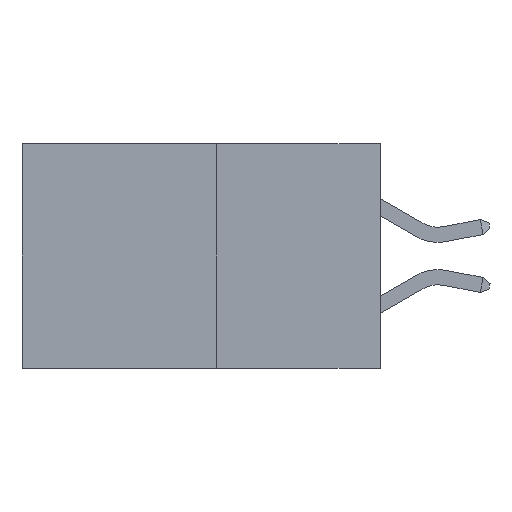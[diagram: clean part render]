
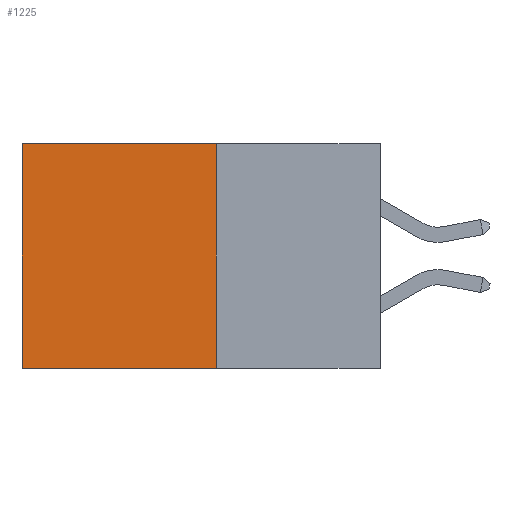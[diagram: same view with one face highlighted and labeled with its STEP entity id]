
A CAD part, left-side view. The second image highlights one B-rep face of the part: STEP entity #1225.
In plain terms, the highlighted planar face has unit normal (-1, 0, 0).
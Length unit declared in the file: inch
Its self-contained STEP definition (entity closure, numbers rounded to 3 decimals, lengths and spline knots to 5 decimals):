
#675 = CARTESIAN_POINT ( 'NONE',  ( 0.277, 0.59, -0.37 ) ) ;
#767 = LINE ( 'NONE', #675, #10291 ) ;
#862 = CARTESIAN_POINT ( 'NONE',  ( 0.277, 0.59, -0.37 ) ) ;
#999 = DIRECTION ( 'NONE',  ( 0., 1., 0. ) ) ;
#1225 = ADVANCED_FACE ( 'NONE', ( #3927 ), #4560, .F. ) ;
#1863 = CARTESIAN_POINT ( 'NONE',  ( 0.277, 0.27, 0. ) ) ;
#2005 = LINE ( 'NONE', #7385, #6738 ) ;
#2748 = LINE ( 'NONE', #10388, #7497 ) ;
#3927 = FACE_OUTER_BOUND ( 'NONE', #4762, .T. ) ;
#4355 = EDGE_CURVE ( 'NONE', #11208, #12252, #2748, .T. ) ;
#4516 = VECTOR ( 'NONE', #7399, 39.37008 ) ;
#4560 = PLANE ( 'NONE',  #9421 ) ;
#4762 = EDGE_LOOP ( 'NONE', ( #5655, #6199, #12001, #10567 ) ) ;
#5626 = CARTESIAN_POINT ( 'NONE',  ( 0.277, 0.59, 0. ) ) ;
#5655 = ORIENTED_EDGE ( 'NONE', *, *, #9495, .T. ) ;
#6199 = ORIENTED_EDGE ( 'NONE', *, *, #4355, .F. ) ;
#6327 = DIRECTION ( 'NONE',  ( 0., 0., -1. ) ) ;
#6738 = VECTOR ( 'NONE', #7334, 39.37008 ) ;
#7334 = DIRECTION ( 'NONE',  ( 0., 0., -1. ) ) ;
#7385 = CARTESIAN_POINT ( 'NONE',  ( 0.277, 0.27, -0.37 ) ) ;
#7399 = DIRECTION ( 'NONE',  ( 0., 1., 0. ) ) ;
#7424 = CARTESIAN_POINT ( 'NONE',  ( 0.277, 0.27, 0. ) ) ;
#7497 = VECTOR ( 'NONE', #999, 39.37008 ) ;
#8087 = EDGE_CURVE ( 'NONE', #10358, #9649, #9901, .T. ) ;
#8111 = EDGE_CURVE ( 'NONE', #10358, #11208, #2005, .T. ) ;
#9421 = AXIS2_PLACEMENT_3D ( 'NONE', #11756, #12106, #11628 ) ;
#9495 = EDGE_CURVE ( 'NONE', #9649, #12252, #767, .T. ) ;
#9649 = VERTEX_POINT ( 'NONE', #5626 ) ;
#9756 = CARTESIAN_POINT ( 'NONE',  ( 0.277, 0.27, -0.37 ) ) ;
#9901 = LINE ( 'NONE', #7424, #4516 ) ;
#10291 = VECTOR ( 'NONE', #6327, 39.37008 ) ;
#10358 = VERTEX_POINT ( 'NONE', #1863 ) ;
#10388 = CARTESIAN_POINT ( 'NONE',  ( 0.277, 0.27, -0.37 ) ) ;
#10567 = ORIENTED_EDGE ( 'NONE', *, *, #8087, .T. ) ;
#11208 = VERTEX_POINT ( 'NONE', #9756 ) ;
#11628 = DIRECTION ( 'NONE',  ( 0., 0., -1. ) ) ;
#11756 = CARTESIAN_POINT ( 'NONE',  ( 0.277, 0.27, -0.37 ) ) ;
#12001 = ORIENTED_EDGE ( 'NONE', *, *, #8111, .F. ) ;
#12106 = DIRECTION ( 'NONE',  ( 1., 0., 0. ) ) ;
#12252 = VERTEX_POINT ( 'NONE', #862 ) ;
